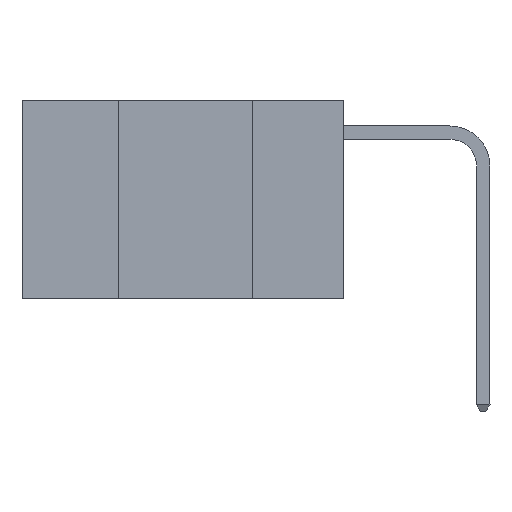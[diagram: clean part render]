
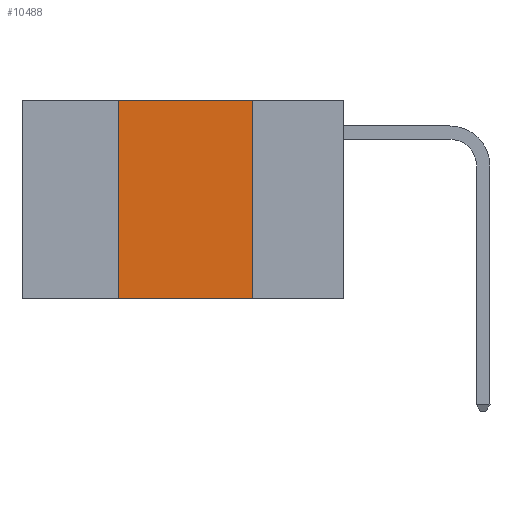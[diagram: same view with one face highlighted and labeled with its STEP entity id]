
A CAD part, left-side view. The second image highlights one B-rep face of the part: STEP entity #10488.
In plain terms, the highlighted planar face has unit normal (-1, 0, 0).
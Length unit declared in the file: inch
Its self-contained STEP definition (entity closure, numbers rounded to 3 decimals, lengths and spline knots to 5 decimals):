
#559 = VECTOR ( 'NONE', #8591, 39.37008 ) ;
#696 = ORIENTED_EDGE ( 'NONE', *, *, #2507, .F. ) ;
#809 = ORIENTED_EDGE ( 'NONE', *, *, #2357, .F. ) ;
#951 = CARTESIAN_POINT ( 'NONE',  ( 0., 0.6, 0. ) ) ;
#1081 = EDGE_CURVE ( 'NONE', #12381, #12481, #7224, .T. ) ;
#1153 = CARTESIAN_POINT ( 'NONE',  ( 0., 0.42, 0. ) ) ;
#1393 = CARTESIAN_POINT ( 'NONE',  ( 0., 0.6, -0.37 ) ) ;
#1759 = DIRECTION ( 'NONE',  ( 0., -1., 0. ) ) ;
#1884 = EDGE_CURVE ( 'NONE', #12381, #6651, #7786, .T. ) ;
#1939 = DIRECTION ( 'NONE',  ( 0., 0., 1. ) ) ;
#2009 = DIRECTION ( 'NONE',  ( 1., 0., 0. ) ) ;
#2357 = EDGE_CURVE ( 'NONE', #7123, #6651, #8639, .T. ) ;
#2507 = EDGE_CURVE ( 'NONE', #12481, #7123, #7038, .T. ) ;
#2720 = CARTESIAN_POINT ( 'NONE',  ( 0., 0.17, 0. ) ) ;
#2724 = VECTOR ( 'NONE', #12792, 39.37008 ) ;
#3065 = DIRECTION ( 'NONE',  ( 0., 0., -1. ) ) ;
#3751 = CARTESIAN_POINT ( 'NONE',  ( 0., 0.6, 0. ) ) ;
#5230 = VECTOR ( 'NONE', #1939, 39.37008 ) ;
#6117 = ORIENTED_EDGE ( 'NONE', *, *, #1884, .T. ) ;
#6380 = FACE_OUTER_BOUND ( 'NONE', #10337, .T. ) ;
#6651 = VERTEX_POINT ( 'NONE', #10354 ) ;
#7038 = LINE ( 'NONE', #3751, #7650 ) ;
#7123 = VERTEX_POINT ( 'NONE', #2720 ) ;
#7224 = LINE ( 'NONE', #1153, #5230 ) ;
#7650 = VECTOR ( 'NONE', #1759, 39.37008 ) ;
#7786 = LINE ( 'NONE', #1393, #559 ) ;
#8347 = PLANE ( 'NONE',  #8741 ) ;
#8591 = DIRECTION ( 'NONE',  ( 0., -1., 0. ) ) ;
#8639 = LINE ( 'NONE', #12657, #2724 ) ;
#8741 = AXIS2_PLACEMENT_3D ( 'NONE', #951, #2009, #3065 ) ;
#9561 = CARTESIAN_POINT ( 'NONE',  ( 0., 0.42, 0. ) ) ;
#10337 = EDGE_LOOP ( 'NONE', ( #809, #696, #11541, #6117 ) ) ;
#10354 = CARTESIAN_POINT ( 'NONE',  ( 0., 0.17, -0.37 ) ) ;
#10488 = ADVANCED_FACE ( 'NONE', ( #6380 ), #8347, .F. ) ;
#10491 = CARTESIAN_POINT ( 'NONE',  ( 0., 0.42, -0.37 ) ) ;
#11541 = ORIENTED_EDGE ( 'NONE', *, *, #1081, .F. ) ;
#12381 = VERTEX_POINT ( 'NONE', #10491 ) ;
#12481 = VERTEX_POINT ( 'NONE', #9561 ) ;
#12657 = CARTESIAN_POINT ( 'NONE',  ( 0., 0.17, 0. ) ) ;
#12792 = DIRECTION ( 'NONE',  ( 0., 0., -1. ) ) ;
